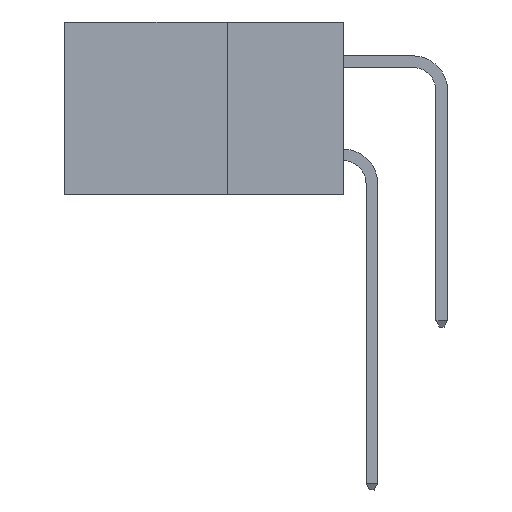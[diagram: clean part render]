
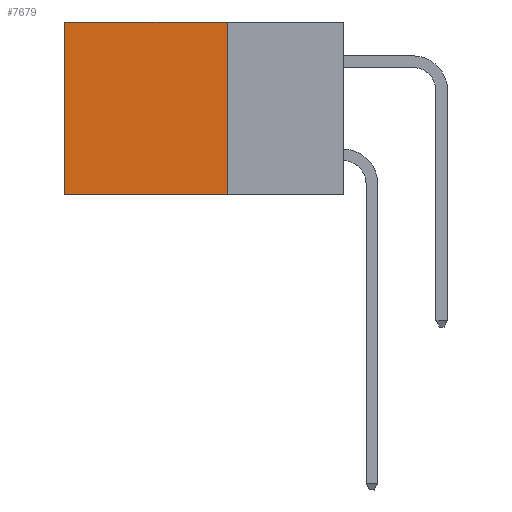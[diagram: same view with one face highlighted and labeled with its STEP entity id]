
A CAD part, left-side view. The second image highlights one B-rep face of the part: STEP entity #7679.
In plain terms, the highlighted planar face has unit normal (-1, 0, 0).
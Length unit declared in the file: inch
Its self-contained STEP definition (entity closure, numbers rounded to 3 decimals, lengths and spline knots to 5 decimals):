
#322 = DIRECTION ( 'NONE',  ( 0., 1., 0. ) ) ;
#529 = CARTESIAN_POINT ( 'NONE',  ( 0.298, 0.25, 0. ) ) ;
#619 = CARTESIAN_POINT ( 'NONE',  ( 0.298, 0.25, -0.37 ) ) ;
#1414 = ORIENTED_EDGE ( 'NONE', *, *, #18890, .F. ) ;
#1756 = EDGE_CURVE ( 'NONE', #20221, #4466, #15690, .T. ) ;
#1926 = CARTESIAN_POINT ( 'NONE',  ( 0.298, 0.25, 0. ) ) ;
#2356 = DIRECTION ( 'NONE',  ( 0., 0., -1. ) ) ;
#3679 = ORIENTED_EDGE ( 'NONE', *, *, #20998, .F. ) ;
#4094 = LINE ( 'NONE', #7846, #17543 ) ;
#4466 = VERTEX_POINT ( 'NONE', #14389 ) ;
#5016 = LINE ( 'NONE', #529, #13898 ) ;
#6034 = EDGE_LOOP ( 'NONE', ( #17079, #1414, #3679, #16920 ) ) ;
#7264 = VERTEX_POINT ( 'NONE', #18251 ) ;
#7679 = ADVANCED_FACE ( 'NONE', ( #17884 ), #19415, .F. ) ;
#7846 = CARTESIAN_POINT ( 'NONE',  ( 0.298, 0.6, 0. ) ) ;
#9270 = DIRECTION ( 'NONE',  ( 0., 1., 0. ) ) ;
#9309 = CARTESIAN_POINT ( 'NONE',  ( 0.298, 0.25, 0. ) ) ;
#9681 = DIRECTION ( 'NONE',  ( 0., 0., -1. ) ) ;
#10440 = VERTEX_POINT ( 'NONE', #619 ) ;
#10869 = DIRECTION ( 'NONE',  ( 0., 0., -1. ) ) ;
#11914 = AXIS2_PLACEMENT_3D ( 'NONE', #16017, #21086, #10869 ) ;
#13486 = VECTOR ( 'NONE', #9270, 39.37008 ) ;
#13898 = VECTOR ( 'NONE', #2356, 39.37008 ) ;
#14025 = LINE ( 'NONE', #14461, #13486 ) ;
#14389 = CARTESIAN_POINT ( 'NONE',  ( 0.298, 0.6, 0. ) ) ;
#14461 = CARTESIAN_POINT ( 'NONE',  ( 0.298, 0.25, -0.37 ) ) ;
#15690 = LINE ( 'NONE', #9309, #16763 ) ;
#16017 = CARTESIAN_POINT ( 'NONE',  ( 0.298, 0.25, 0. ) ) ;
#16763 = VECTOR ( 'NONE', #322, 39.37008 ) ;
#16920 = ORIENTED_EDGE ( 'NONE', *, *, #1756, .T. ) ;
#17079 = ORIENTED_EDGE ( 'NONE', *, *, #18509, .T. ) ;
#17543 = VECTOR ( 'NONE', #9681, 39.37008 ) ;
#17884 = FACE_OUTER_BOUND ( 'NONE', #6034, .T. ) ;
#18251 = CARTESIAN_POINT ( 'NONE',  ( 0.298, 0.6, -0.37 ) ) ;
#18509 = EDGE_CURVE ( 'NONE', #4466, #7264, #4094, .T. ) ;
#18890 = EDGE_CURVE ( 'NONE', #10440, #7264, #14025, .T. ) ;
#19415 = PLANE ( 'NONE',  #11914 ) ;
#20221 = VERTEX_POINT ( 'NONE', #1926 ) ;
#20998 = EDGE_CURVE ( 'NONE', #20221, #10440, #5016, .T. ) ;
#21086 = DIRECTION ( 'NONE',  ( 1., 0., 0. ) ) ;
